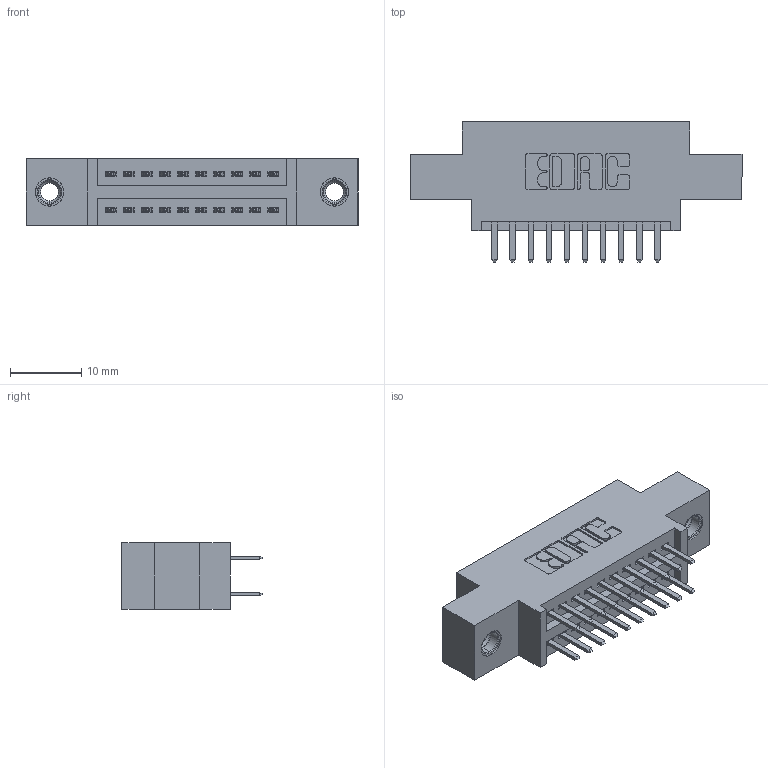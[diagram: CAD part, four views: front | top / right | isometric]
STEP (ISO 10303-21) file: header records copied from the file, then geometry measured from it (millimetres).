
FILE_DESCRIPTION (( 'STEP AP203' ), '1' );
FILE_NAME ('395-020-520-807.STEP', '2019-10-15T20:47:22', ( '' ), ( '' ), 'SwSTEP 2.0', 'SolidWorks 2016', '' );
FILE_SCHEMA (( 'CONFIG_CONTROL_DESIGN' ));
Length unit declared in the file: inch
Products named in the file (4): 345 Part_0.170 Offset - 0.156 Dia-TI; 345-292-001_345-293-120; 345-250-001_345-250-005-103; 395-020-520-807
Assembly tree (23 placements, depth 2):
  395-020-520-807
    345 Part_0.170 Offset - 0.156 Dia-TI
    345-292-001_345-293-120  x20
    345-250-001_345-250-005-103  x2
Bounding box: 46.61 x 19.68 x 9.4 mm (x, y, z)
Volume: 4094.9 mm3; surface area: 5585.9 mm2
Topology: 23 solids, 23 shells, 1270 faces, 3629 edges, 2358 vertices
Faces by surface type: plane 816, cylinder 438, cone 12, torus 4
Entity records: 13586 total; most frequent: CARTESIAN_POINT 2303, ORIENTED_EDGE 2218, DIRECTION 2083, EDGE_CURVE 1109, VECTOR 913, LINE 913, VERTEX_POINT 732, AXIS2_PLACEMENT_3D 585
